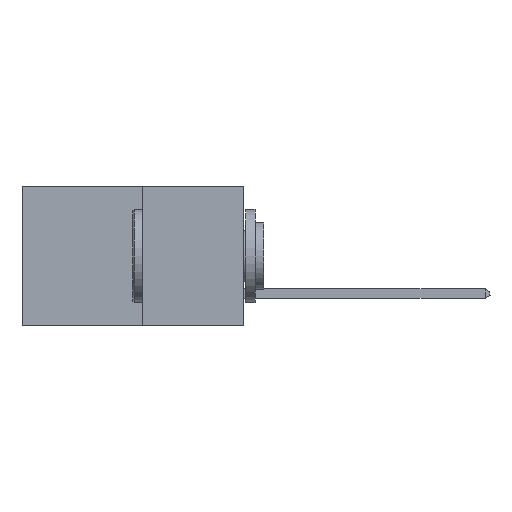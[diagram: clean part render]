
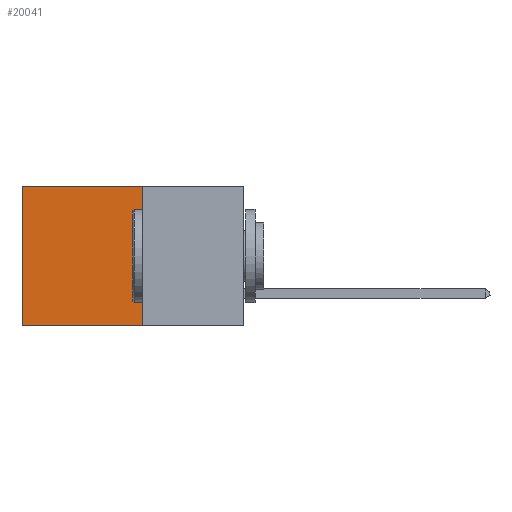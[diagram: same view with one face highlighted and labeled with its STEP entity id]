
A CAD part, left-side view. The second image highlights one B-rep face of the part: STEP entity #20041.
In plain terms, the highlighted planar face has unit normal (-1, 0, 0).
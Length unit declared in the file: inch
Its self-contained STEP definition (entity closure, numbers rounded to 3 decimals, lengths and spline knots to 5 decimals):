
#146 = CARTESIAN_POINT ( 'NONE',  ( 0.277, 0.27, -0.37 ) ) ;
#1353 = CARTESIAN_POINT ( 'NONE',  ( 0.277, 0.27, -0.37 ) ) ;
#1485 = LINE ( 'NONE', #21878, #13281 ) ;
#1951 = EDGE_CURVE ( 'NONE', #5313, #14135, #3655, .T. ) ;
#2235 = FACE_OUTER_BOUND ( 'NONE', #13945, .T. ) ;
#2487 = DIRECTION ( 'NONE',  ( 0., 1., 0. ) ) ;
#2656 = DIRECTION ( 'NONE',  ( 0., 1., 0. ) ) ;
#3345 = CARTESIAN_POINT ( 'NONE',  ( 0.277, 0.27, -0.37 ) ) ;
#3655 = LINE ( 'NONE', #3345, #22261 ) ;
#3681 = DIRECTION ( 'NONE',  ( 0., 0., -1. ) ) ;
#4666 = LINE ( 'NONE', #146, #17124 ) ;
#5143 = CARTESIAN_POINT ( 'NONE',  ( 0.277, 0.27, 0. ) ) ;
#5313 = VERTEX_POINT ( 'NONE', #5143 ) ;
#7289 = ORIENTED_EDGE ( 'NONE', *, *, #17797, .F. ) ;
#7651 = ORIENTED_EDGE ( 'NONE', *, *, #28105, .T. ) ;
#8441 = EDGE_CURVE ( 'NONE', #5313, #12063, #12022, .T. ) ;
#8447 = DIRECTION ( 'NONE',  ( 1., 0., 0. ) ) ;
#9471 = CARTESIAN_POINT ( 'NONE',  ( 0.277, 0.59, 0. ) ) ;
#10095 = CARTESIAN_POINT ( 'NONE',  ( 0.277, 0.27, -0.37 ) ) ;
#10749 = PLANE ( 'NONE',  #29269 ) ;
#12022 = LINE ( 'NONE', #23550, #29674 ) ;
#12063 = VERTEX_POINT ( 'NONE', #9471 ) ;
#12437 = ORIENTED_EDGE ( 'NONE', *, *, #8441, .T. ) ;
#12992 = VERTEX_POINT ( 'NONE', #20095 ) ;
#13180 = ORIENTED_EDGE ( 'NONE', *, *, #1951, .F. ) ;
#13281 = VECTOR ( 'NONE', #28795, 39.37008 ) ;
#13945 = EDGE_LOOP ( 'NONE', ( #7651, #7289, #13180, #12437 ) ) ;
#14135 = VERTEX_POINT ( 'NONE', #10095 ) ;
#17124 = VECTOR ( 'NONE', #2487, 39.37008 ) ;
#17797 = EDGE_CURVE ( 'NONE', #14135, #12992, #4666, .T. ) ;
#20041 = ADVANCED_FACE ( 'NONE', ( #2235 ), #10749, .F. ) ;
#20095 = CARTESIAN_POINT ( 'NONE',  ( 0.277, 0.59, -0.37 ) ) ;
#21878 = CARTESIAN_POINT ( 'NONE',  ( 0.277, 0.59, -0.37 ) ) ;
#22261 = VECTOR ( 'NONE', #3681, 39.37008 ) ;
#23550 = CARTESIAN_POINT ( 'NONE',  ( 0.277, 0.27, 0. ) ) ;
#24665 = DIRECTION ( 'NONE',  ( 0., 0., -1. ) ) ;
#28105 = EDGE_CURVE ( 'NONE', #12063, #12992, #1485, .T. ) ;
#28795 = DIRECTION ( 'NONE',  ( 0., 0., -1. ) ) ;
#29269 = AXIS2_PLACEMENT_3D ( 'NONE', #1353, #8447, #24665 ) ;
#29674 = VECTOR ( 'NONE', #2656, 39.37008 ) ;
